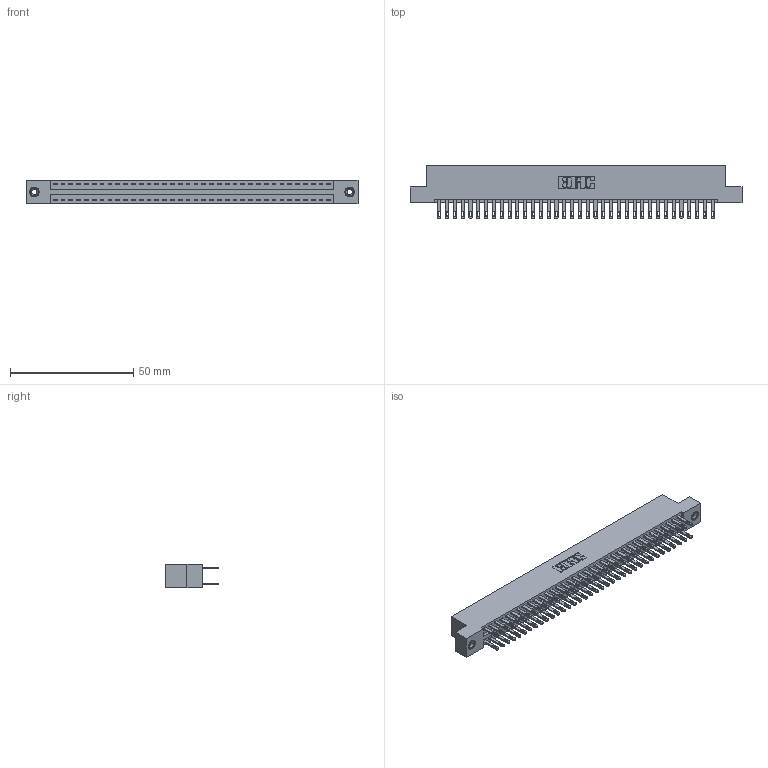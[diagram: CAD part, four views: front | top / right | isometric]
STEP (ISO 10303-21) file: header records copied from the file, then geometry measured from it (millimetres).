
FILE_DESCRIPTION (( 'STEP AP203' ), '1' );
FILE_NAME ('896-072-500-208.STEP', '2021-07-28T01:23:08', ( '' ), ( '' ), 'SwSTEP 2.0', 'SolidWorks 2020', '' );
FILE_SCHEMA (( 'CONFIG_CONTROL_DESIGN' ));
Length unit declared in the file: inch
Products named in the file (4): 345-292-001_345-293-100; 345-250-001_345-250-003-102; 846 Part_Flush Mounting Lugs - 0.156 Dia-TI; 896-072-500-208
Assembly tree (75 placements, depth 2):
  896-072-500-208
    846 Part_Flush Mounting Lugs - 0.156 Dia-TI
    345-292-001_345-293-100  x72
    345-250-001_345-250-003-102  x2
Bounding box: 134.87 x 21.84 x 9.4 mm (x, y, z)
Volume: 13318.8 mm3; surface area: 18986.9 mm2
Topology: 75 solids, 75 shells, 3638 faces, 11049 edges, 7358 vertices
Faces by surface type: plane 2196, cylinder 1426, cone 12, torus 4
Entity records: 25418 total; most frequent: CARTESIAN_POINT 4179, ORIENTED_EDGE 4106, DIRECTION 3763, EDGE_CURVE 2053, LINE 1753, VECTOR 1753, VERTEX_POINT 1364, AXIS2_PLACEMENT_3D 1005
